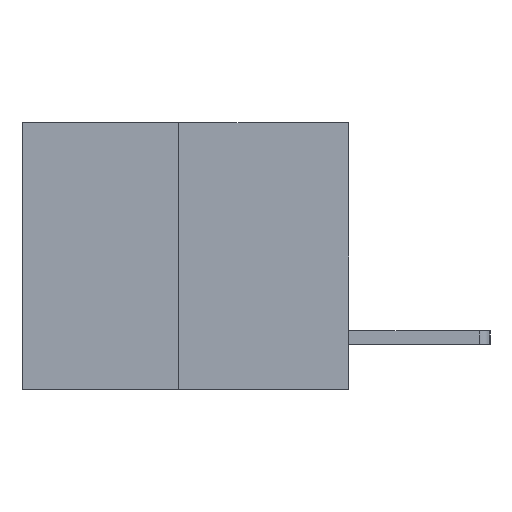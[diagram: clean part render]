
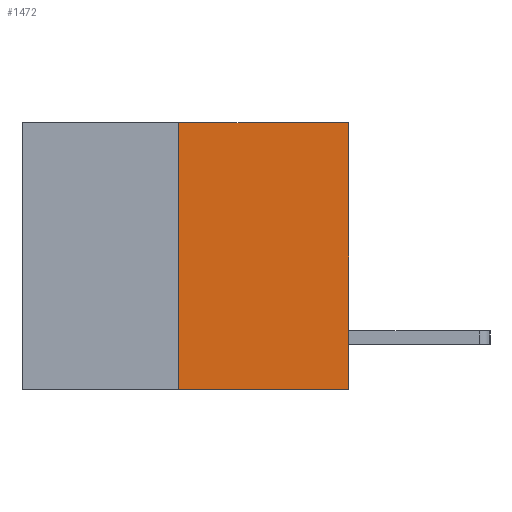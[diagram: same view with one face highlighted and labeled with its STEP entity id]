
A CAD part, left-side view. The second image highlights one B-rep face of the part: STEP entity #1472.
In plain terms, the highlighted planar face has unit normal (-1, 0, 0).
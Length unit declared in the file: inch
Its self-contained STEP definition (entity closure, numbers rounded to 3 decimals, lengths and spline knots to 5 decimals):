
#35 = PLANE ( 'NONE',  #9155 ) ;
#210 = VECTOR ( 'NONE', #7208, 39.37008 ) ;
#349 = CARTESIAN_POINT ( 'NONE',  ( 0., 0.6, -0.49 ) ) ;
#480 = ORIENTED_EDGE ( 'NONE', *, *, #7114, .F. ) ;
#1162 = DIRECTION ( 'NONE',  ( 0., -1., 0. ) ) ;
#1204 = ORIENTED_EDGE ( 'NONE', *, *, #9448, .T. ) ;
#1472 = ADVANCED_FACE ( 'NONE', ( #5480 ), #35, .F. ) ;
#1643 = CARTESIAN_POINT ( 'NONE',  ( 0., 0., -0.49 ) ) ;
#1960 = CARTESIAN_POINT ( 'NONE',  ( 0., 0.6, 0. ) ) ;
#2568 = CARTESIAN_POINT ( 'NONE',  ( 0., 0.312, -0.49 ) ) ;
#3173 = VECTOR ( 'NONE', #5182, 39.37008 ) ;
#3759 = CARTESIAN_POINT ( 'NONE',  ( 0., 0.312, -0.49 ) ) ;
#4248 = LINE ( 'NONE', #3759, #210 ) ;
#4726 = VERTEX_POINT ( 'NONE', #6087 ) ;
#5000 = LINE ( 'NONE', #9212, #5653 ) ;
#5182 = DIRECTION ( 'NONE',  ( 0., -1., 0. ) ) ;
#5415 = LINE ( 'NONE', #6971, #3173 ) ;
#5480 = FACE_OUTER_BOUND ( 'NONE', #7530, .T. ) ;
#5653 = VECTOR ( 'NONE', #10881, 39.37008 ) ;
#5983 = CARTESIAN_POINT ( 'NONE',  ( 0., 0., 0. ) ) ;
#6087 = CARTESIAN_POINT ( 'NONE',  ( 0., 0.312, 0. ) ) ;
#6126 = VERTEX_POINT ( 'NONE', #2568 ) ;
#6567 = ORIENTED_EDGE ( 'NONE', *, *, #6955, .T. ) ;
#6712 = DIRECTION ( 'NONE',  ( 0., 0., -1. ) ) ;
#6955 = EDGE_CURVE ( 'NONE', #6126, #7376, #9326, .T. ) ;
#6971 = CARTESIAN_POINT ( 'NONE',  ( 0., 0.6, 0. ) ) ;
#7114 = EDGE_CURVE ( 'NONE', #6126, #4726, #4248, .T. ) ;
#7208 = DIRECTION ( 'NONE',  ( 0., 0., 1. ) ) ;
#7376 = VERTEX_POINT ( 'NONE', #1643 ) ;
#7530 = EDGE_LOOP ( 'NONE', ( #480, #6567, #1204, #8502 ) ) ;
#7878 = VECTOR ( 'NONE', #1162, 39.37008 ) ;
#8229 = EDGE_CURVE ( 'NONE', #4726, #8959, #5415, .T. ) ;
#8502 = ORIENTED_EDGE ( 'NONE', *, *, #8229, .F. ) ;
#8959 = VERTEX_POINT ( 'NONE', #5983 ) ;
#9155 = AXIS2_PLACEMENT_3D ( 'NONE', #1960, #10069, #6712 ) ;
#9212 = CARTESIAN_POINT ( 'NONE',  ( 0., 0., 0. ) ) ;
#9326 = LINE ( 'NONE', #349, #7878 ) ;
#9448 = EDGE_CURVE ( 'NONE', #7376, #8959, #5000, .T. ) ;
#10069 = DIRECTION ( 'NONE',  ( 1., 0., 0. ) ) ;
#10881 = DIRECTION ( 'NONE',  ( 0., 0., 1. ) ) ;
